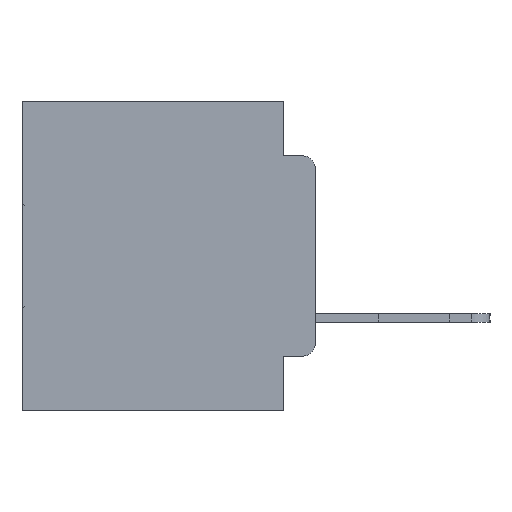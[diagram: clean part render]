
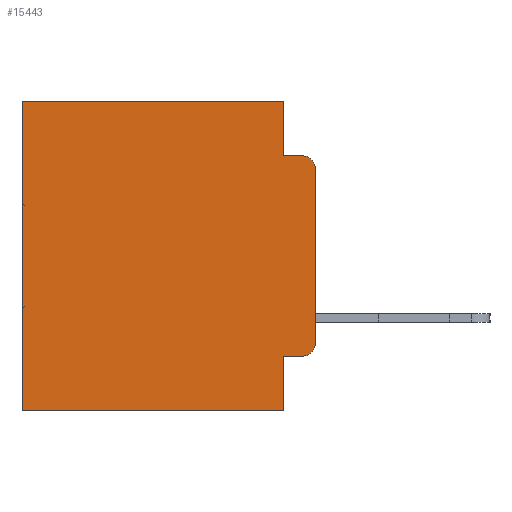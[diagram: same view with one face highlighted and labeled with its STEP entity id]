
A CAD part, left-side view. The second image highlights one B-rep face of the part: STEP entity #15443.
In plain terms, the highlighted planar face has unit normal (-1, 0, 0).
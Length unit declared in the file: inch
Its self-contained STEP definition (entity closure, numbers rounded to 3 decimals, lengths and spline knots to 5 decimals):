
#279 = EDGE_CURVE ( 'NONE', #20576, #10525, #18064, .T. ) ;
#893 = DIRECTION ( 'NONE',  ( 0., 1., 0. ) ) ;
#1921 = EDGE_CURVE ( 'NONE', #28477, #7639, #19396, .T. ) ;
#2104 = DIRECTION ( 'NONE',  ( 0., -1., 0. ) ) ;
#2321 = DIRECTION ( 'NONE',  ( 0., 0., -1. ) ) ;
#2447 = ORIENTED_EDGE ( 'NONE', *, *, #4422, .T. ) ;
#2888 = FACE_OUTER_BOUND ( 'NONE', #20786, .T. ) ;
#2930 = CARTESIAN_POINT ( 'NONE',  ( 0.298, 0.051, -0.5 ) ) ;
#3995 = ORIENTED_EDGE ( 'NONE', *, *, #9439, .T. ) ;
#4139 = VERTEX_POINT ( 'NONE', #5423 ) ;
#4422 = EDGE_CURVE ( 'NONE', #28477, #23133, #24002, .T. ) ;
#4467 = VECTOR ( 'NONE', #7068, 39.37008 ) ;
#4660 = DIRECTION ( 'NONE',  ( 0., 0., -1. ) ) ;
#4981 = DIRECTION ( 'NONE',  ( 0., 0., -1. ) ) ;
#5053 = DIRECTION ( 'NONE',  ( 0., 0., -1. ) ) ;
#5366 = CARTESIAN_POINT ( 'NONE',  ( 0.298, 0.051, 0. ) ) ;
#5423 = CARTESIAN_POINT ( 'NONE',  ( 0.298, 0.473, 0. ) ) ;
#5472 = EDGE_CURVE ( 'NONE', #4139, #22530, #16030, .T. ) ;
#6880 = AXIS2_PLACEMENT_3D ( 'NONE', #30841, #16950, #2321 ) ;
#7025 = CARTESIAN_POINT ( 'NONE',  ( 0.298, 0., 0. ) ) ;
#7068 = DIRECTION ( 'NONE',  ( 0., 0., -1. ) ) ;
#7485 = ORIENTED_EDGE ( 'NONE', *, *, #16301, .F. ) ;
#7639 = VERTEX_POINT ( 'NONE', #2930 ) ;
#8098 = EDGE_CURVE ( 'NONE', #23133, #10525, #18740, .T. ) ;
#8144 = CARTESIAN_POINT ( 'NONE',  ( 0.298, 0.051, 0. ) ) ;
#8186 = ORIENTED_EDGE ( 'NONE', *, *, #279, .F. ) ;
#9439 = EDGE_CURVE ( 'NONE', #20576, #19577, #19543, .T. ) ;
#9633 = CARTESIAN_POINT ( 'NONE',  ( 0.298, 0.051, -0.4115 ) ) ;
#9817 = VECTOR ( 'NONE', #4660, 39.37008 ) ;
#9825 = CARTESIAN_POINT ( 'NONE',  ( 0.298, 0., 0. ) ) ;
#9978 = VERTEX_POINT ( 'NONE', #19704 ) ;
#10146 = DIRECTION ( 'NONE',  ( 0., 1., 0. ) ) ;
#10525 = VERTEX_POINT ( 'NONE', #17167 ) ;
#10811 = CARTESIAN_POINT ( 'NONE',  ( 0.298, 0.02, -0.0885 ) ) ;
#11729 = ORIENTED_EDGE ( 'NONE', *, *, #1921, .F. ) ;
#11909 = CARTESIAN_POINT ( 'NONE',  ( 0.298, 0.473, -0.5 ) ) ;
#11969 = LINE ( 'NONE', #26579, #24384 ) ;
#12136 = ORIENTED_EDGE ( 'NONE', *, *, #8098, .T. ) ;
#12341 = EDGE_CURVE ( 'NONE', #9978, #19577, #29590, .T. ) ;
#12869 = DIRECTION ( 'NONE',  ( -1., 0., 0. ) ) ;
#13224 = CARTESIAN_POINT ( 'NONE',  ( 0.298, 0., -0.1085 ) ) ;
#13983 = VECTOR ( 'NONE', #20583, 39.37008 ) ;
#14484 = CARTESIAN_POINT ( 'NONE',  ( 0.298, 0.473, 0. ) ) ;
#15443 = ADVANCED_FACE ( 'NONE', ( #2888 ), #17069, .F. ) ;
#15629 = VERTEX_POINT ( 'NONE', #8144 ) ;
#15836 = ORIENTED_EDGE ( 'NONE', *, *, #5472, .T. ) ;
#16030 = LINE ( 'NONE', #14484, #26163 ) ;
#16233 = LINE ( 'NONE', #25947, #9817 ) ;
#16301 = EDGE_CURVE ( 'NONE', #7639, #22530, #26709, .T. ) ;
#16950 = DIRECTION ( 'NONE',  ( -1., 0., 0. ) ) ;
#17069 = PLANE ( 'NONE',  #29155 ) ;
#17167 = CARTESIAN_POINT ( 'NONE',  ( 0.298, 0., -0.3915 ) ) ;
#18009 = CARTESIAN_POINT ( 'NONE',  ( 0.298, 0., -0.5 ) ) ;
#18064 = LINE ( 'NONE', #7025, #4467 ) ;
#18076 = EDGE_CURVE ( 'NONE', #15629, #4139, #11969, .T. ) ;
#18354 = ORIENTED_EDGE ( 'NONE', *, *, #24126, .F. ) ;
#18690 = DIRECTION ( 'NONE',  ( 0., -1., 0. ) ) ;
#18740 = CIRCLE ( 'NONE', #6880, 0.02 ) ;
#19369 = DIRECTION ( 'NONE',  ( 1., 0., 0. ) ) ;
#19396 = LINE ( 'NONE', #5366, #13983 ) ;
#19543 = CIRCLE ( 'NONE', #22074, 0.02 ) ;
#19577 = VERTEX_POINT ( 'NONE', #10811 ) ;
#19704 = CARTESIAN_POINT ( 'NONE',  ( 0.298, 0.051, -0.0885 ) ) ;
#19783 = VECTOR ( 'NONE', #893, 39.37008 ) ;
#20576 = VERTEX_POINT ( 'NONE', #13224 ) ;
#20583 = DIRECTION ( 'NONE',  ( 0., 0., -1. ) ) ;
#20786 = EDGE_LOOP ( 'NONE', ( #8186, #3995, #28576, #18354, #25963, #15836, #7485, #11729, #2447, #12136 ) ) ;
#22074 = AXIS2_PLACEMENT_3D ( 'NONE', #26815, #12869, #29187 ) ;
#22530 = VERTEX_POINT ( 'NONE', #11909 ) ;
#22648 = VECTOR ( 'NONE', #2104, 39.37008 ) ;
#23133 = VERTEX_POINT ( 'NONE', #30648 ) ;
#24002 = LINE ( 'NONE', #9633, #25445 ) ;
#24126 = EDGE_CURVE ( 'NONE', #15629, #9978, #16233, .T. ) ;
#24384 = VECTOR ( 'NONE', #10146, 39.37008 ) ;
#25445 = VECTOR ( 'NONE', #18690, 39.37008 ) ;
#25947 = CARTESIAN_POINT ( 'NONE',  ( 0.298, 0.051, 0. ) ) ;
#25963 = ORIENTED_EDGE ( 'NONE', *, *, #18076, .T. ) ;
#26163 = VECTOR ( 'NONE', #5053, 39.37008 ) ;
#26579 = CARTESIAN_POINT ( 'NONE',  ( 0.298, 0., 0. ) ) ;
#26709 = LINE ( 'NONE', #18009, #19783 ) ;
#26815 = CARTESIAN_POINT ( 'NONE',  ( 0.298, 0.02, -0.1085 ) ) ;
#26938 = CARTESIAN_POINT ( 'NONE',  ( 0.298, 0.051, -0.4115 ) ) ;
#28477 = VERTEX_POINT ( 'NONE', #26938 ) ;
#28576 = ORIENTED_EDGE ( 'NONE', *, *, #12341, .F. ) ;
#29155 = AXIS2_PLACEMENT_3D ( 'NONE', #9825, #19369, #4981 ) ;
#29187 = DIRECTION ( 'NONE',  ( 0., 0., -1. ) ) ;
#29590 = LINE ( 'NONE', #30660, #22648 ) ;
#30648 = CARTESIAN_POINT ( 'NONE',  ( 0.298, 0.02, -0.4115 ) ) ;
#30660 = CARTESIAN_POINT ( 'NONE',  ( 0.298, 0.051, -0.0885 ) ) ;
#30841 = CARTESIAN_POINT ( 'NONE',  ( 0.298, 0.02, -0.3915 ) ) ;
